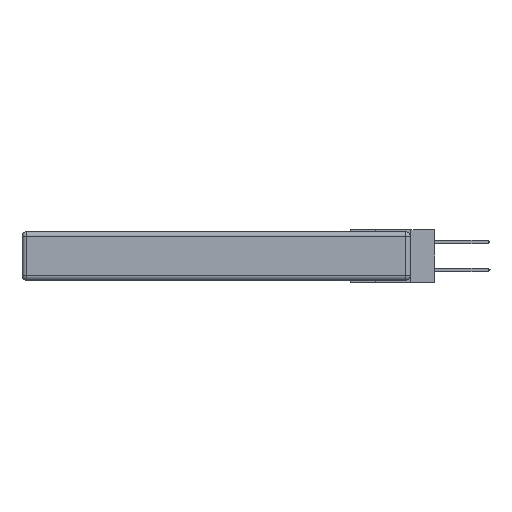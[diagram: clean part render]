
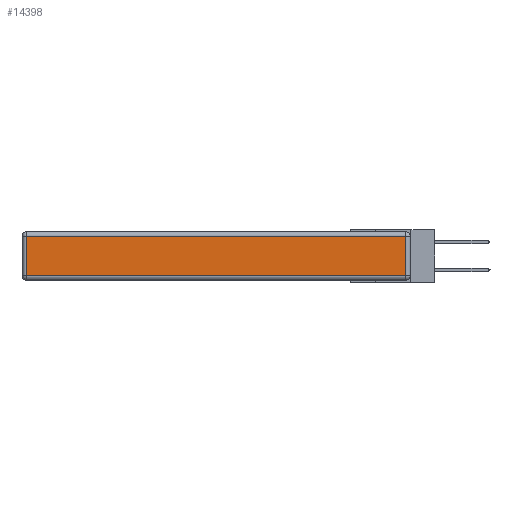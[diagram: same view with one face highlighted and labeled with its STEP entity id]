
A CAD part, left-side view. The second image highlights one B-rep face of the part: STEP entity #14398.
In plain terms, the highlighted planar face has unit normal (-1, 0, 0).
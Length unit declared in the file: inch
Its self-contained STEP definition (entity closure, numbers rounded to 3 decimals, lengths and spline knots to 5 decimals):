
#677 = LINE ( 'NONE', #10168, #13027 ) ;
#828 = VERTEX_POINT ( 'NONE', #3159 ) ;
#1041 = EDGE_LOOP ( 'NONE', ( #7122, #15942, #14274, #4271 ) ) ;
#1321 = VECTOR ( 'NONE', #8171, 39.37008 ) ;
#2119 = DIRECTION ( 'NONE',  ( 0., 1., 0. ) ) ;
#2129 = LINE ( 'NONE', #4393, #1321 ) ;
#2579 = EDGE_CURVE ( 'NONE', #16711, #6934, #8374, .T. ) ;
#2862 = CARTESIAN_POINT ( 'NONE',  ( 0., 0.03, -0.03 ) ) ;
#3059 = CARTESIAN_POINT ( 'NONE',  ( 0., 0.03, -0.343 ) ) ;
#3159 = CARTESIAN_POINT ( 'NONE',  ( 0., 2.72, -0.313 ) ) ;
#4271 = ORIENTED_EDGE ( 'NONE', *, *, #8802, .T. ) ;
#4393 = CARTESIAN_POINT ( 'NONE',  ( 0., 2.72, -0.343 ) ) ;
#4553 = CARTESIAN_POINT ( 'NONE',  ( 0., 0., -0.343 ) ) ;
#5495 = DIRECTION ( 'NONE',  ( 0., 0., 1. ) ) ;
#5702 = CARTESIAN_POINT ( 'NONE',  ( 0., 2.75, -0.03 ) ) ;
#6201 = LINE ( 'NONE', #5702, #15456 ) ;
#6934 = VERTEX_POINT ( 'NONE', #2862 ) ;
#7122 = ORIENTED_EDGE ( 'NONE', *, *, #9494, .T. ) ;
#8171 = DIRECTION ( 'NONE',  ( 0., 0., -1. ) ) ;
#8374 = LINE ( 'NONE', #3059, #14750 ) ;
#8390 = VERTEX_POINT ( 'NONE', #11291 ) ;
#8802 = EDGE_CURVE ( 'NONE', #8390, #828, #2129, .T. ) ;
#9494 = EDGE_CURVE ( 'NONE', #828, #16711, #677, .T. ) ;
#10111 = DIRECTION ( 'NONE',  ( 0., 0., 1. ) ) ;
#10168 = CARTESIAN_POINT ( 'NONE',  ( 0., 0., -0.313 ) ) ;
#11291 = CARTESIAN_POINT ( 'NONE',  ( 0., 2.72, -0.03 ) ) ;
#11489 = DIRECTION ( 'NONE',  ( 0., -1., 0. ) ) ;
#11858 = FACE_OUTER_BOUND ( 'NONE', #1041, .T. ) ;
#11908 = AXIS2_PLACEMENT_3D ( 'NONE', #4553, #16672, #10111 ) ;
#13027 = VECTOR ( 'NONE', #11489, 39.37008 ) ;
#14274 = ORIENTED_EDGE ( 'NONE', *, *, #14941, .T. ) ;
#14398 = ADVANCED_FACE ( 'NONE', ( #11858 ), #16147, .T. ) ;
#14673 = CARTESIAN_POINT ( 'NONE',  ( 0., 0.03, -0.313 ) ) ;
#14750 = VECTOR ( 'NONE', #5495, 39.37008 ) ;
#14941 = EDGE_CURVE ( 'NONE', #6934, #8390, #6201, .T. ) ;
#15456 = VECTOR ( 'NONE', #2119, 39.37008 ) ;
#15942 = ORIENTED_EDGE ( 'NONE', *, *, #2579, .T. ) ;
#16147 = PLANE ( 'NONE',  #11908 ) ;
#16672 = DIRECTION ( 'NONE',  ( -1., 0., 0. ) ) ;
#16711 = VERTEX_POINT ( 'NONE', #14673 ) ;
